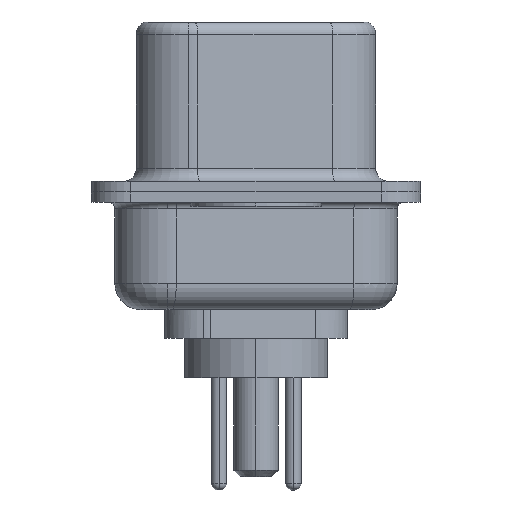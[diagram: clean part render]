
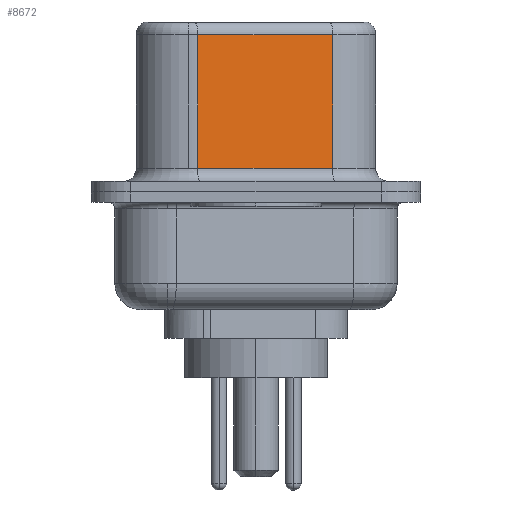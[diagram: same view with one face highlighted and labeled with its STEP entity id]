
A CAD part, left-side view. The second image highlights one B-rep face of the part: STEP entity #8672.
In plain terms, the highlighted planar face has unit normal (-0.985, -0.174, 0).
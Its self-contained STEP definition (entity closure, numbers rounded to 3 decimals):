
#251 = VECTOR ( 'NONE', #380, 1000. ) ;
#380 = DIRECTION ( 'NONE',  ( 0., 0., -1. ) ) ;
#1146 = VERTEX_POINT ( 'NONE', #13415 ) ;
#1479 = LINE ( 'NONE', #15484, #11697 ) ;
#1524 = ORIENTED_EDGE ( 'NONE', *, *, #8398, .T. ) ;
#1811 = VERTEX_POINT ( 'NONE', #4088 ) ;
#1845 = DIRECTION ( 'NONE',  ( 0.174, -0.985, 0. ) ) ;
#1920 = DIRECTION ( 'NONE',  ( -0.174, 0.985, 0. ) ) ;
#2565 = DIRECTION ( 'NONE',  ( 0., 0., -1. ) ) ;
#2583 = EDGE_CURVE ( 'NONE', #16181, #1146, #3966, .T. ) ;
#2751 = VECTOR ( 'NONE', #2565, 1000. ) ;
#3023 = FACE_OUTER_BOUND ( 'NONE', #13916, .T. ) ;
#3492 = AXIS2_PLACEMENT_3D ( 'NONE', #13488, #17108, #10850 ) ;
#3655 = EDGE_CURVE ( 'NONE', #16181, #1811, #1479, .T. ) ;
#3827 = LINE ( 'NONE', #16573, #251 ) ;
#3966 = LINE ( 'NONE', #11735, #2751 ) ;
#4088 = CARTESIAN_POINT ( 'NONE',  ( 3.675, 2.233, 6.02 ) ) ;
#4730 = ORIENTED_EDGE ( 'NONE', *, *, #12343, .T. ) ;
#6623 = VERTEX_POINT ( 'NONE', #11223 ) ;
#7379 = CARTESIAN_POINT ( 'NONE',  ( 4.585, -2.927, 0.9 ) ) ;
#8398 = EDGE_CURVE ( 'NONE', #6623, #1146, #13730, .T. ) ;
#8672 = ADVANCED_FACE ( 'NONE', ( #3023 ), #13100, .F. ) ;
#10682 = CARTESIAN_POINT ( 'NONE',  ( 4.585, -2.927, 6.02 ) ) ;
#10850 = DIRECTION ( 'NONE',  ( -0.174, 0.985, 0. ) ) ;
#11097 = ORIENTED_EDGE ( 'NONE', *, *, #3655, .T. ) ;
#11223 = CARTESIAN_POINT ( 'NONE',  ( 3.675, 2.233, 0.9 ) ) ;
#11697 = VECTOR ( 'NONE', #1920, 1000. ) ;
#11735 = CARTESIAN_POINT ( 'NONE',  ( 4.585, -2.927, 6.52 ) ) ;
#12343 = EDGE_CURVE ( 'NONE', #1811, #6623, #3827, .T. ) ;
#13100 = PLANE ( 'NONE',  #3492 ) ;
#13270 = VECTOR ( 'NONE', #1845, 1000. ) ;
#13415 = CARTESIAN_POINT ( 'NONE',  ( 4.585, -2.927, 0.9 ) ) ;
#13488 = CARTESIAN_POINT ( 'NONE',  ( 4.585, -2.927, 6.52 ) ) ;
#13730 = LINE ( 'NONE', #7379, #13270 ) ;
#13916 = EDGE_LOOP ( 'NONE', ( #15267, #11097, #4730, #1524 ) ) ;
#15267 = ORIENTED_EDGE ( 'NONE', *, *, #2583, .F. ) ;
#15484 = CARTESIAN_POINT ( 'NONE',  ( 4.585, -2.927, 6.02 ) ) ;
#16181 = VERTEX_POINT ( 'NONE', #10682 ) ;
#16573 = CARTESIAN_POINT ( 'NONE',  ( 3.675, 2.233, 6.52 ) ) ;
#17108 = DIRECTION ( 'NONE',  ( 0.985, 0.174, 0. ) ) ;
